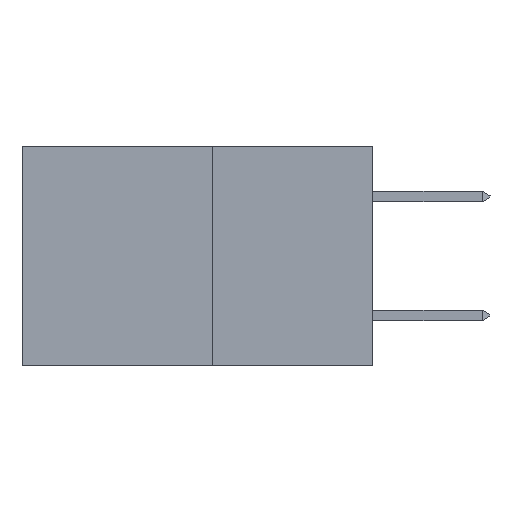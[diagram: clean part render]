
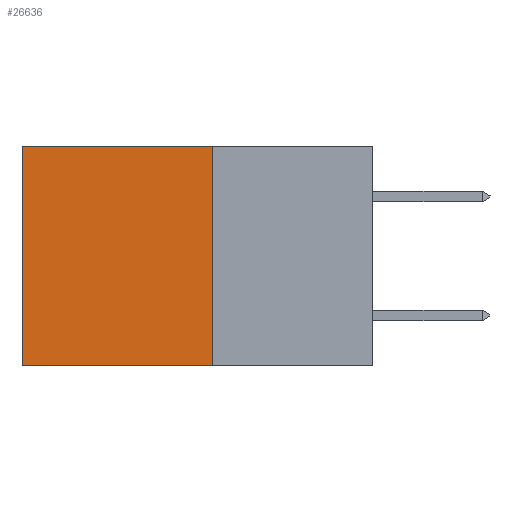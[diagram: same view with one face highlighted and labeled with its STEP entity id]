
A CAD part, left-side view. The second image highlights one B-rep face of the part: STEP entity #26636.
In plain terms, the highlighted planar face has unit normal (-1, 0, 0).
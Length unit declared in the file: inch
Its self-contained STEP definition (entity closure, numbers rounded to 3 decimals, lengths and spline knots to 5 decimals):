
#12 = EDGE_CURVE ( 'NONE', #15365, #10336, #4886, .T. ) ;
#236 = DIRECTION ( 'NONE',  ( 0., 0., -1. ) ) ;
#1485 = ORIENTED_EDGE ( 'NONE', *, *, #27422, .F. ) ;
#1600 = CARTESIAN_POINT ( 'NONE',  ( 0.277, 0.59, -0.37 ) ) ;
#1955 = VECTOR ( 'NONE', #2019, 39.37008 ) ;
#2019 = DIRECTION ( 'NONE',  ( 0., 1., 0. ) ) ;
#4886 = LINE ( 'NONE', #23816, #32705 ) ;
#5749 = CARTESIAN_POINT ( 'NONE',  ( 0.277, 0.27, -0.37 ) ) ;
#6652 = LINE ( 'NONE', #5749, #26483 ) ;
#6990 = CARTESIAN_POINT ( 'NONE',  ( 0.277, 0.27, -0.37 ) ) ;
#9130 = LINE ( 'NONE', #28763, #1955 ) ;
#9731 = DIRECTION ( 'NONE',  ( 0., 0., -1. ) ) ;
#9948 = AXIS2_PLACEMENT_3D ( 'NONE', #6990, #25863, #9731 ) ;
#10336 = VERTEX_POINT ( 'NONE', #13915 ) ;
#10722 = DIRECTION ( 'NONE',  ( 0., 0., -1. ) ) ;
#11407 = EDGE_CURVE ( 'NONE', #15365, #14269, #6652, .T. ) ;
#11498 = DIRECTION ( 'NONE',  ( 0., 1., 0. ) ) ;
#13915 = CARTESIAN_POINT ( 'NONE',  ( 0.277, 0.59, 0. ) ) ;
#14269 = VERTEX_POINT ( 'NONE', #19013 ) ;
#15365 = VERTEX_POINT ( 'NONE', #34860 ) ;
#17556 = ORIENTED_EDGE ( 'NONE', *, *, #11407, .F. ) ;
#19013 = CARTESIAN_POINT ( 'NONE',  ( 0.277, 0.27, -0.37 ) ) ;
#19631 = LINE ( 'NONE', #21813, #31414 ) ;
#20032 = VERTEX_POINT ( 'NONE', #1600 ) ;
#21076 = ORIENTED_EDGE ( 'NONE', *, *, #22334, .T. ) ;
#21813 = CARTESIAN_POINT ( 'NONE',  ( 0.277, 0.59, -0.37 ) ) ;
#22334 = EDGE_CURVE ( 'NONE', #10336, #20032, #19631, .T. ) ;
#23145 = PLANE ( 'NONE',  #9948 ) ;
#23816 = CARTESIAN_POINT ( 'NONE',  ( 0.277, 0.27, 0. ) ) ;
#25863 = DIRECTION ( 'NONE',  ( 1., 0., 0. ) ) ;
#26483 = VECTOR ( 'NONE', #10722, 39.37008 ) ;
#26636 = ADVANCED_FACE ( 'NONE', ( #32815 ), #23145, .F. ) ;
#27422 = EDGE_CURVE ( 'NONE', #14269, #20032, #9130, .T. ) ;
#28763 = CARTESIAN_POINT ( 'NONE',  ( 0.277, 0.27, -0.37 ) ) ;
#31414 = VECTOR ( 'NONE', #236, 39.37008 ) ;
#32705 = VECTOR ( 'NONE', #11498, 39.37008 ) ;
#32815 = FACE_OUTER_BOUND ( 'NONE', #34168, .T. ) ;
#33407 = ORIENTED_EDGE ( 'NONE', *, *, #12, .T. ) ;
#34168 = EDGE_LOOP ( 'NONE', ( #21076, #1485, #17556, #33407 ) ) ;
#34860 = CARTESIAN_POINT ( 'NONE',  ( 0.277, 0.27, 0. ) ) ;
